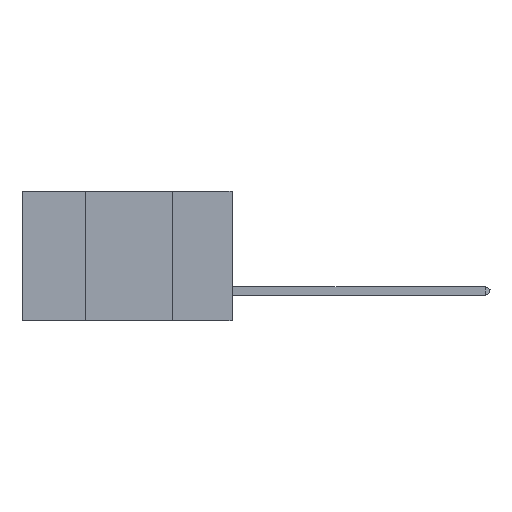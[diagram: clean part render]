
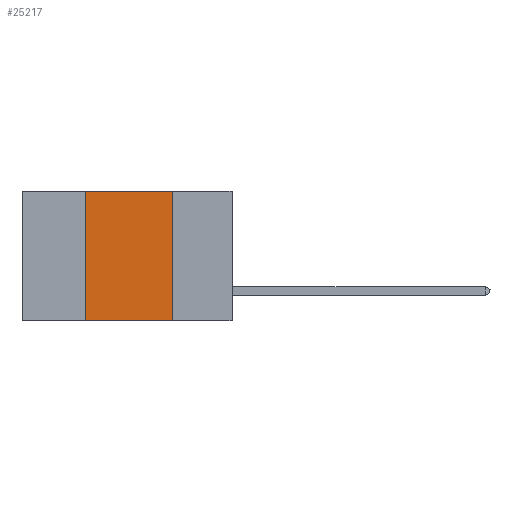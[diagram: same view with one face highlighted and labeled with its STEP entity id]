
A CAD part, left-side view. The second image highlights one B-rep face of the part: STEP entity #25217.
In plain terms, the highlighted planar face has unit normal (-1, 0, 0).
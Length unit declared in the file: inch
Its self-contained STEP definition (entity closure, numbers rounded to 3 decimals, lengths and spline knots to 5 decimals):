
#407 = VECTOR ( 'NONE', #28973, 39.37008 ) ;
#417 = DIRECTION ( 'NONE',  ( 0., -1., 0. ) ) ;
#679 = CARTESIAN_POINT ( 'NONE',  ( 0., 0.6, 0. ) ) ;
#3793 = CARTESIAN_POINT ( 'NONE',  ( 0., 0.6, 0. ) ) ;
#3977 = DIRECTION ( 'NONE',  ( 0., 0., -1. ) ) ;
#4581 = VERTEX_POINT ( 'NONE', #30804 ) ;
#4981 = CARTESIAN_POINT ( 'NONE',  ( 0., 0.6, -0.37 ) ) ;
#6930 = ORIENTED_EDGE ( 'NONE', *, *, #19704, .T. ) ;
#8631 = CARTESIAN_POINT ( 'NONE',  ( 0., 0.42, -0.37 ) ) ;
#9753 = EDGE_LOOP ( 'NONE', ( #29232, #39721, #27641, #6930 ) ) ;
#11452 = VECTOR ( 'NONE', #3977, 39.37008 ) ;
#11645 = FACE_OUTER_BOUND ( 'NONE', #9753, .T. ) ;
#14602 = LINE ( 'NONE', #4981, #33110 ) ;
#18242 = CARTESIAN_POINT ( 'NONE',  ( 0., 0.42, 0. ) ) ;
#19055 = DIRECTION ( 'NONE',  ( 1., 0., 0. ) ) ;
#19584 = LINE ( 'NONE', #679, #35130 ) ;
#19704 = EDGE_CURVE ( 'NONE', #23382, #4581, #14602, .T. ) ;
#21679 = VERTEX_POINT ( 'NONE', #18242 ) ;
#21945 = EDGE_CURVE ( 'NONE', #23382, #21679, #37269, .T. ) ;
#23382 = VERTEX_POINT ( 'NONE', #8631 ) ;
#25217 = ADVANCED_FACE ( 'NONE', ( #11645 ), #31443, .F. ) ;
#25512 = VERTEX_POINT ( 'NONE', #36380 ) ;
#25855 = CARTESIAN_POINT ( 'NONE',  ( 0., 0.42, 0. ) ) ;
#27641 = ORIENTED_EDGE ( 'NONE', *, *, #21945, .F. ) ;
#28894 = CARTESIAN_POINT ( 'NONE',  ( 0., 0.17, 0. ) ) ;
#28973 = DIRECTION ( 'NONE',  ( 0., 0., 1. ) ) ;
#29232 = ORIENTED_EDGE ( 'NONE', *, *, #34679, .F. ) ;
#29819 = EDGE_CURVE ( 'NONE', #21679, #25512, #19584, .T. ) ;
#30804 = CARTESIAN_POINT ( 'NONE',  ( 0., 0.17, -0.37 ) ) ;
#31443 = PLANE ( 'NONE',  #32695 ) ;
#32345 = LINE ( 'NONE', #28894, #11452 ) ;
#32695 = AXIS2_PLACEMENT_3D ( 'NONE', #3793, #19055, #37945 ) ;
#32892 = DIRECTION ( 'NONE',  ( 0., -1., 0. ) ) ;
#33110 = VECTOR ( 'NONE', #32892, 39.37008 ) ;
#34679 = EDGE_CURVE ( 'NONE', #25512, #4581, #32345, .T. ) ;
#35130 = VECTOR ( 'NONE', #417, 39.37008 ) ;
#36380 = CARTESIAN_POINT ( 'NONE',  ( 0., 0.17, 0. ) ) ;
#37269 = LINE ( 'NONE', #25855, #407 ) ;
#37945 = DIRECTION ( 'NONE',  ( 0., 0., -1. ) ) ;
#39721 = ORIENTED_EDGE ( 'NONE', *, *, #29819, .F. ) ;
